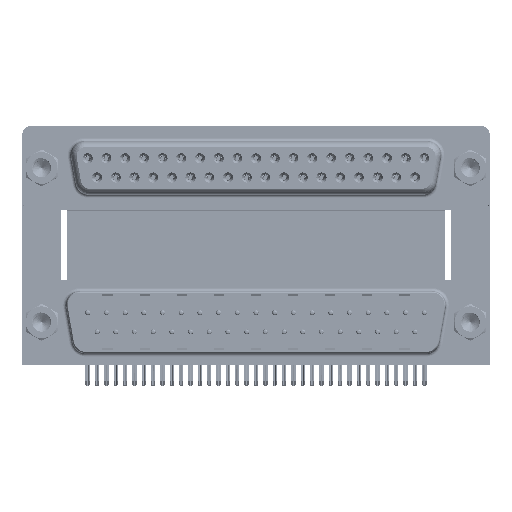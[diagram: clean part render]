
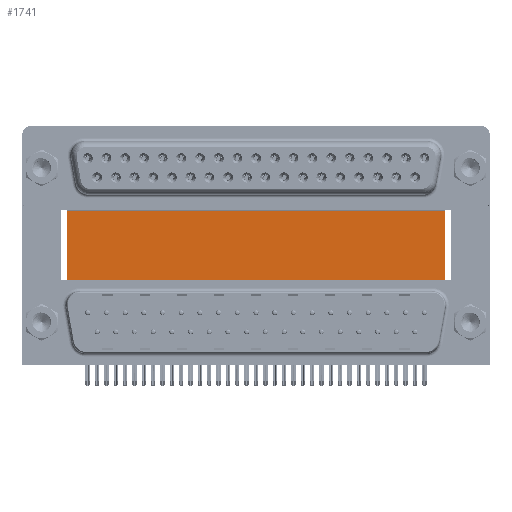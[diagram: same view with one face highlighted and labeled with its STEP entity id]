
A CAD part, top view. The second image highlights one B-rep face of the part: STEP entity #1741.
In plain terms, the highlighted planar face has unit normal (0, 0, 1).
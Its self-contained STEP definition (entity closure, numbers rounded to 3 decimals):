
#1741 = ADVANCED_FACE ( 'NONE', ( #57562 ), #46566, .F. ) ;
#2906 = ORIENTED_EDGE ( 'NONE', *, *, #49693, .F. ) ;
#3716 = CARTESIAN_POINT ( 'NONE',  ( 59.71, 16.585, -12. ) ) ;
#4898 = LINE ( 'NONE', #33507, #29413 ) ;
#6622 = ORIENTED_EDGE ( 'NONE', *, *, #40919, .F. ) ;
#8275 = CARTESIAN_POINT ( 'NONE',  ( 59.71, -3.735, -12. ) ) ;
#11953 = AXIS2_PLACEMENT_3D ( 'NONE', #68938, #68191, #35936 ) ;
#16798 = CARTESIAN_POINT ( 'NONE',  ( 3.79, -3.735, -12. ) ) ;
#17914 = CARTESIAN_POINT ( 'NONE',  ( 3.79, 16.585, -12. ) ) ;
#27836 = VERTEX_POINT ( 'NONE', #16798 ) ;
#29239 = DIRECTION ( 'NONE',  ( 0., -1., 0. ) ) ;
#29413 = VECTOR ( 'NONE', #71654, 1000. ) ;
#31612 = ORIENTED_EDGE ( 'NONE', *, *, #50895, .T. ) ;
#33507 = CARTESIAN_POINT ( 'NONE',  ( 3.79, 16.585, -12. ) ) ;
#35936 = DIRECTION ( 'NONE',  ( -1., 0., 0. ) ) ;
#37225 = EDGE_CURVE ( 'NONE', #71745, #27836, #4898, .T. ) ;
#37308 = ORIENTED_EDGE ( 'NONE', *, *, #37225, .T. ) ;
#37432 = VECTOR ( 'NONE', #29239, 1000. ) ;
#38968 = VERTEX_POINT ( 'NONE', #3716 ) ;
#39510 = CARTESIAN_POINT ( 'NONE',  ( 59.71, 16.585, -12. ) ) ;
#39525 = DIRECTION ( 'NONE',  ( 1., 0., 0. ) ) ;
#40919 = EDGE_CURVE ( 'NONE', #71745, #38968, #42903, .T. ) ;
#42903 = LINE ( 'NONE', #65277, #64773 ) ;
#43247 = DIRECTION ( 'NONE',  ( 1., 0., 0. ) ) ;
#46566 = PLANE ( 'NONE',  #11953 ) ;
#49693 = EDGE_CURVE ( 'NONE', #38968, #65465, #57111, .T. ) ;
#50521 = CARTESIAN_POINT ( 'NONE',  ( 3.79, -3.735, -12. ) ) ;
#50895 = EDGE_CURVE ( 'NONE', #27836, #65465, #57495, .T. ) ;
#57111 = LINE ( 'NONE', #39510, #37432 ) ;
#57495 = LINE ( 'NONE', #50521, #60928 ) ;
#57562 = FACE_OUTER_BOUND ( 'NONE', #63686, .T. ) ;
#60928 = VECTOR ( 'NONE', #39525, 1000. ) ;
#63686 = EDGE_LOOP ( 'NONE', ( #31612, #2906, #6622, #37308 ) ) ;
#64773 = VECTOR ( 'NONE', #43247, 1000. ) ;
#65277 = CARTESIAN_POINT ( 'NONE',  ( 3.79, 16.585, -12. ) ) ;
#65465 = VERTEX_POINT ( 'NONE', #8275 ) ;
#68191 = DIRECTION ( 'NONE',  ( 0., 0., -1. ) ) ;
#68938 = CARTESIAN_POINT ( 'NONE',  ( 3.79, 16.585, -12. ) ) ;
#71654 = DIRECTION ( 'NONE',  ( 0., -1., 0. ) ) ;
#71745 = VERTEX_POINT ( 'NONE', #17914 ) ;
